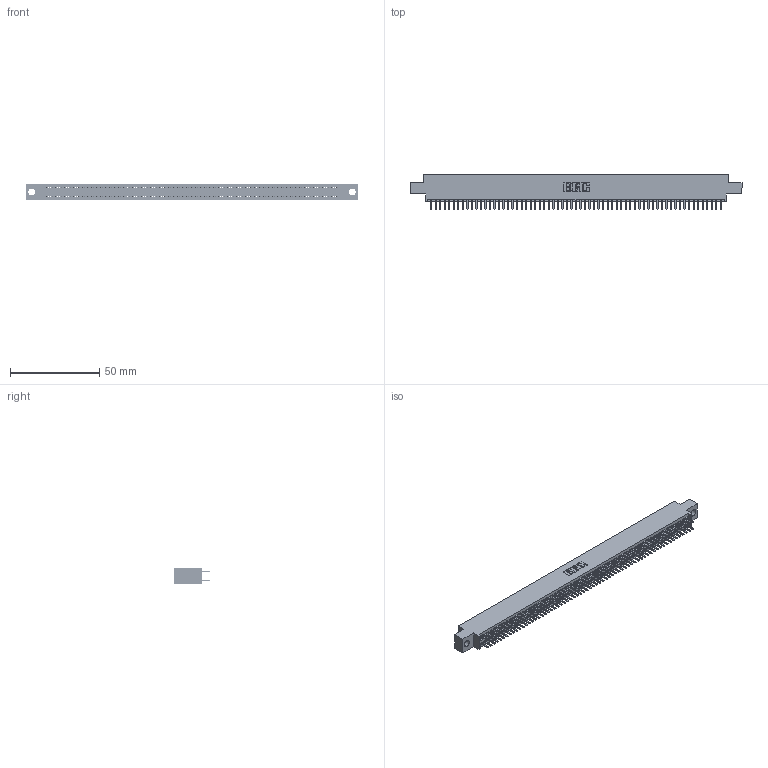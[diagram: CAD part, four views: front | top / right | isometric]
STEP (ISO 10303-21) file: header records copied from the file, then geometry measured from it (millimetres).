
FILE_DESCRIPTION (( 'STEP AP203' ), '1' );
FILE_NAME ('345-130-520-804.STEP', '2018-10-19T23:06:48', ( '' ), ( '' ), 'SwSTEP 2.0', 'SolidWorks 2016', '' );
FILE_SCHEMA (( 'CONFIG_CONTROL_DESIGN' ));
Length unit declared in the file: inch
Products named in the file (3): 345-292-001_345-293-120; 345-130-520-804; 345 Part_0.170 Offset - 0.156 Dia-TH
Assembly tree (131 placements, depth 2):
  345-130-520-804
    345 Part_0.170 Offset - 0.156 Dia-TH
    345-292-001_345-293-120  x130
Bounding box: 186.31 x 19.68 x 9.4 mm (x, y, z)
Volume: 18053.3 mm3; surface area: 26968.4 mm2
Topology: 131 solids, 131 shells, 7150 faces, 20763 edges, 13494 vertices
Faces by surface type: plane 4634, cylinder 2516
Entity records: 48153 total; most frequent: CARTESIAN_POINT 8064, ORIENTED_EDGE 7986, DIRECTION 7069, EDGE_CURVE 3993, VECTOR 3597, LINE 3597, VERTEX_POINT 2658, AXIS2_PLACEMENT_3D 1736
